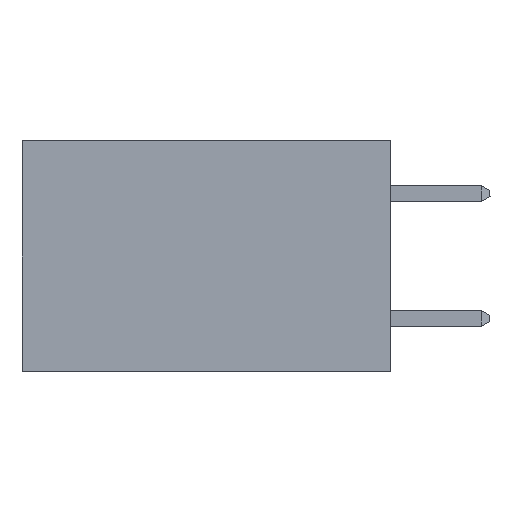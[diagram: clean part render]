
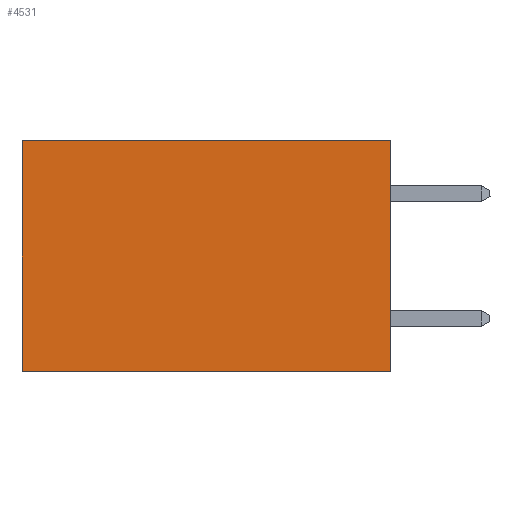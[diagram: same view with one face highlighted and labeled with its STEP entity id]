
A CAD part, left-side view. The second image highlights one B-rep face of the part: STEP entity #4531.
In plain terms, the highlighted planar face has unit normal (-1, 0, 0).
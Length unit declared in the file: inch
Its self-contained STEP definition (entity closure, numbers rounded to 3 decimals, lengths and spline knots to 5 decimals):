
#187 = LINE ( 'NONE', #27344, #27221 ) ;
#215 = CARTESIAN_POINT ( 'NONE',  ( 0.277, 0., 0. ) ) ;
#1557 = CARTESIAN_POINT ( 'NONE',  ( 0.277, 0.59, 0. ) ) ;
#3427 = EDGE_CURVE ( 'NONE', #4262, #28149, #16038, .T. ) ;
#3625 = CARTESIAN_POINT ( 'NONE',  ( 0.277, 0.59, -0.37 ) ) ;
#4023 = AXIS2_PLACEMENT_3D ( 'NONE', #8664, #11320, #29585 ) ;
#4262 = VERTEX_POINT ( 'NONE', #23340 ) ;
#4531 = ADVANCED_FACE ( 'NONE', ( #8556 ), #24342, .F. ) ;
#6140 = LINE ( 'NONE', #3625, #19299 ) ;
#6239 = DIRECTION ( 'NONE',  ( 0., 0., -1. ) ) ;
#7740 = DIRECTION ( 'NONE',  ( 0., 1., 0. ) ) ;
#8556 = FACE_OUTER_BOUND ( 'NONE', #31685, .T. ) ;
#8664 = CARTESIAN_POINT ( 'NONE',  ( 0.277, 0., -0.37 ) ) ;
#10413 = ORIENTED_EDGE ( 'NONE', *, *, #24097, .F. ) ;
#11320 = DIRECTION ( 'NONE',  ( 1., 0., 0. ) ) ;
#12488 = EDGE_CURVE ( 'NONE', #33642, #15589, #26518, .T. ) ;
#15589 = VERTEX_POINT ( 'NONE', #1557 ) ;
#16038 = LINE ( 'NONE', #25539, #22168 ) ;
#16943 = ORIENTED_EDGE ( 'NONE', *, *, #3427, .F. ) ;
#16967 = DIRECTION ( 'NONE',  ( 0., 0., -1. ) ) ;
#19299 = VECTOR ( 'NONE', #6239, 39.37008 ) ;
#20118 = EDGE_CURVE ( 'NONE', #15589, #28149, #6140, .T. ) ;
#20809 = CARTESIAN_POINT ( 'NONE',  ( 0.277, 0., 0. ) ) ;
#22168 = VECTOR ( 'NONE', #22940, 39.37008 ) ;
#22940 = DIRECTION ( 'NONE',  ( 0., 1., 0. ) ) ;
#23340 = CARTESIAN_POINT ( 'NONE',  ( 0.277, 0., -0.37 ) ) ;
#24097 = EDGE_CURVE ( 'NONE', #33642, #4262, #187, .T. ) ;
#24342 = PLANE ( 'NONE',  #4023 ) ;
#25539 = CARTESIAN_POINT ( 'NONE',  ( 0.277, 0., -0.37 ) ) ;
#25811 = CARTESIAN_POINT ( 'NONE',  ( 0.277, 0.59, -0.37 ) ) ;
#26155 = ORIENTED_EDGE ( 'NONE', *, *, #20118, .T. ) ;
#26518 = LINE ( 'NONE', #20809, #33454 ) ;
#27221 = VECTOR ( 'NONE', #16967, 39.37008 ) ;
#27344 = CARTESIAN_POINT ( 'NONE',  ( 0.277, 0., -0.37 ) ) ;
#28149 = VERTEX_POINT ( 'NONE', #25811 ) ;
#29585 = DIRECTION ( 'NONE',  ( 0., 0., -1. ) ) ;
#31638 = ORIENTED_EDGE ( 'NONE', *, *, #12488, .T. ) ;
#31685 = EDGE_LOOP ( 'NONE', ( #26155, #16943, #10413, #31638 ) ) ;
#33454 = VECTOR ( 'NONE', #7740, 39.37008 ) ;
#33642 = VERTEX_POINT ( 'NONE', #215 ) ;
